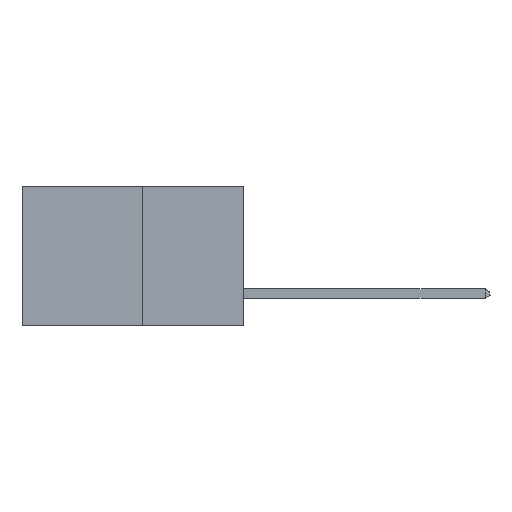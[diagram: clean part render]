
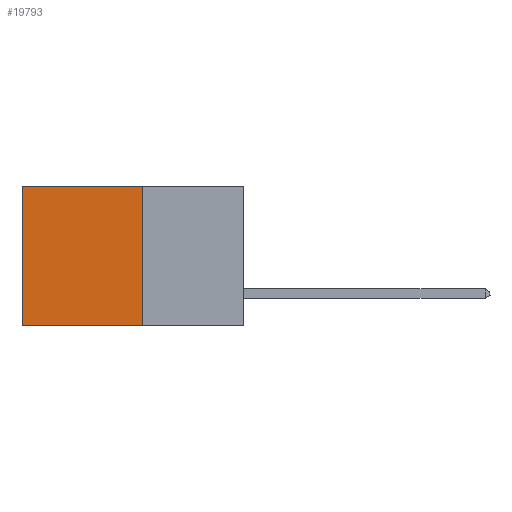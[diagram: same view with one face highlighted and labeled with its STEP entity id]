
A CAD part, left-side view. The second image highlights one B-rep face of the part: STEP entity #19793.
In plain terms, the highlighted planar face has unit normal (-1, 0, 0).
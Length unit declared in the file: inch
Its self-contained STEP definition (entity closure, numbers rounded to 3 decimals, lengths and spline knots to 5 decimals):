
#1168 = CARTESIAN_POINT ( 'NONE',  ( 0.277, 0.59, -0.37 ) ) ;
#1289 = ORIENTED_EDGE ( 'NONE', *, *, #4762, .F. ) ;
#3093 = LINE ( 'NONE', #8923, #28871 ) ;
#4762 = EDGE_CURVE ( 'NONE', #18509, #17505, #7354, .T. ) ;
#5111 = CARTESIAN_POINT ( 'NONE',  ( 0.277, 0.27, -0.37 ) ) ;
#5437 = DIRECTION ( 'NONE',  ( 0., 1., 0. ) ) ;
#7354 = LINE ( 'NONE', #27715, #27056 ) ;
#7912 = CARTESIAN_POINT ( 'NONE',  ( 0.277, 0.27, -0.37 ) ) ;
#8923 = CARTESIAN_POINT ( 'NONE',  ( 0.277, 0.27, -0.37 ) ) ;
#8953 = CARTESIAN_POINT ( 'NONE',  ( 0.277, 0.27, 0. ) ) ;
#9447 = EDGE_LOOP ( 'NONE', ( #14683, #1289, #17174, #31783 ) ) ;
#10312 = DIRECTION ( 'NONE',  ( 1., 0., 0. ) ) ;
#10507 = VERTEX_POINT ( 'NONE', #8953 ) ;
#13294 = CARTESIAN_POINT ( 'NONE',  ( 0.277, 0.59, 0. ) ) ;
#14683 = ORIENTED_EDGE ( 'NONE', *, *, #23979, .T. ) ;
#17174 = ORIENTED_EDGE ( 'NONE', *, *, #23166, .F. ) ;
#17505 = VERTEX_POINT ( 'NONE', #1168 ) ;
#17533 = VECTOR ( 'NONE', #27249, 39.37008 ) ;
#18509 = VERTEX_POINT ( 'NONE', #7912 ) ;
#19793 = ADVANCED_FACE ( 'NONE', ( #32211 ), #20550, .F. ) ;
#20550 = PLANE ( 'NONE',  #25096 ) ;
#23166 = EDGE_CURVE ( 'NONE', #10507, #18509, #3093, .T. ) ;
#23580 = LINE ( 'NONE', #23930, #29555 ) ;
#23930 = CARTESIAN_POINT ( 'NONE',  ( 0.277, 0.27, 0. ) ) ;
#23979 = EDGE_CURVE ( 'NONE', #29711, #17505, #24417, .T. ) ;
#24417 = LINE ( 'NONE', #24674, #17533 ) ;
#24674 = CARTESIAN_POINT ( 'NONE',  ( 0.277, 0.59, -0.37 ) ) ;
#25096 = AXIS2_PLACEMENT_3D ( 'NONE', #5111, #10312, #28291 ) ;
#25300 = DIRECTION ( 'NONE',  ( 0., 1., 0. ) ) ;
#27056 = VECTOR ( 'NONE', #25300, 39.37008 ) ;
#27249 = DIRECTION ( 'NONE',  ( 0., 0., -1. ) ) ;
#27715 = CARTESIAN_POINT ( 'NONE',  ( 0.277, 0.27, -0.37 ) ) ;
#28291 = DIRECTION ( 'NONE',  ( 0., 0., -1. ) ) ;
#28871 = VECTOR ( 'NONE', #32023, 39.37008 ) ;
#29527 = EDGE_CURVE ( 'NONE', #10507, #29711, #23580, .T. ) ;
#29555 = VECTOR ( 'NONE', #5437, 39.37008 ) ;
#29711 = VERTEX_POINT ( 'NONE', #13294 ) ;
#31783 = ORIENTED_EDGE ( 'NONE', *, *, #29527, .T. ) ;
#32023 = DIRECTION ( 'NONE',  ( 0., 0., -1. ) ) ;
#32211 = FACE_OUTER_BOUND ( 'NONE', #9447, .T. ) ;
